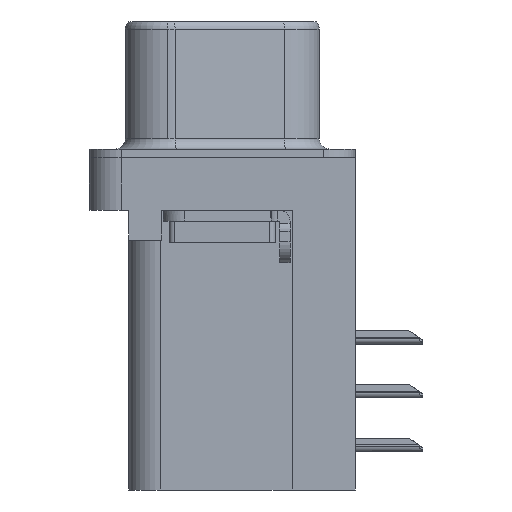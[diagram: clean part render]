
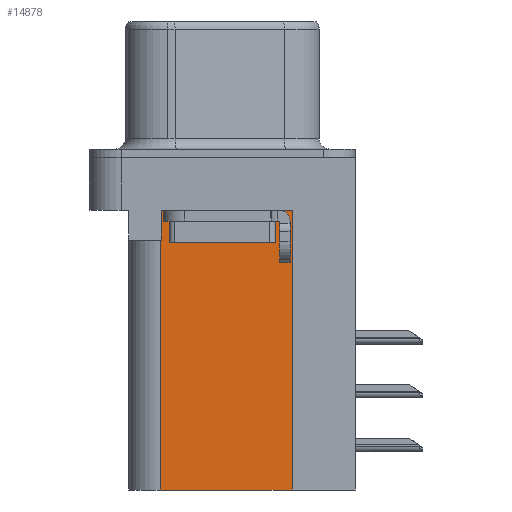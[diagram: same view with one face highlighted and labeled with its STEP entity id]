
A CAD part, left-side view. The second image highlights one B-rep face of the part: STEP entity #14878.
In plain terms, the highlighted planar face has unit normal (-1, 0, 0).
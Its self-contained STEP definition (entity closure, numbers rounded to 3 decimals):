
#390 = CARTESIAN_POINT ( 'NONE',  ( 3.7, -3.295, -15.7 ) ) ;
#563 = CARTESIAN_POINT ( 'NONE',  ( 3.7, -3.295, -15.7 ) ) ;
#1540 = EDGE_CURVE ( 'NONE', #8664, #25485, #20465, .T. ) ;
#1928 = LINE ( 'NONE', #12069, #25458 ) ;
#2034 = ORIENTED_EDGE ( 'NONE', *, *, #10155, .F. ) ;
#2653 = DIRECTION ( 'NONE',  ( 0., 0., -1. ) ) ;
#4221 = ORIENTED_EDGE ( 'NONE', *, *, #1540, .T. ) ;
#5213 = DIRECTION ( 'NONE',  ( 0., 0., 1. ) ) ;
#5603 = EDGE_CURVE ( 'NONE', #20065, #8664, #27021, .T. ) ;
#6796 = LINE ( 'NONE', #17612, #12810 ) ;
#7113 = FACE_OUTER_BOUND ( 'NONE', #16796, .T. ) ;
#8664 = VERTEX_POINT ( 'NONE', #24389 ) ;
#8684 = CARTESIAN_POINT ( 'NONE',  ( 3.7, -3.295, -2.5 ) ) ;
#8689 = DIRECTION ( 'NONE',  ( 0., 1., 0. ) ) ;
#9821 = LINE ( 'NONE', #18837, #22606 ) ;
#10155 = EDGE_CURVE ( 'NONE', #15262, #10890, #9821, .T. ) ;
#10890 = VERTEX_POINT ( 'NONE', #11415 ) ;
#11124 = AXIS2_PLACEMENT_3D ( 'NONE', #390, #16295, #2653 ) ;
#11415 = CARTESIAN_POINT ( 'NONE',  ( 3.7, 2.925, -3.9 ) ) ;
#11631 = CARTESIAN_POINT ( 'NONE',  ( 3.7, 2.895, -3.9 ) ) ;
#12069 = CARTESIAN_POINT ( 'NONE',  ( 3.7, 0., -3.9 ) ) ;
#12181 = EDGE_CURVE ( 'NONE', #12749, #20065, #22903, .T. ) ;
#12749 = VERTEX_POINT ( 'NONE', #28116 ) ;
#12810 = VECTOR ( 'NONE', #20006, 1000. ) ;
#14014 = PLANE ( 'NONE',  #11124 ) ;
#14353 = DIRECTION ( 'NONE',  ( 0., 1., 0. ) ) ;
#14394 = VECTOR ( 'NONE', #25349, 1000. ) ;
#14878 = ADVANCED_FACE ( 'NONE', ( #7113 ), #14014, .F. ) ;
#15262 = VERTEX_POINT ( 'NONE', #19839 ) ;
#16123 = VECTOR ( 'NONE', #25441, 1000. ) ;
#16295 = DIRECTION ( 'NONE',  ( 1., 0., 0. ) ) ;
#16796 = EDGE_LOOP ( 'NONE', ( #21812, #4221, #25150, #2034, #18632, #19967 ) ) ;
#17612 = CARTESIAN_POINT ( 'NONE',  ( 3.7, -3.295, -15.7 ) ) ;
#17690 = CARTESIAN_POINT ( 'NONE',  ( 3.7, -3.295, -2.5 ) ) ;
#18632 = ORIENTED_EDGE ( 'NONE', *, *, #23205, .F. ) ;
#18837 = CARTESIAN_POINT ( 'NONE',  ( 3.7, 2.925, -15.7 ) ) ;
#19839 = CARTESIAN_POINT ( 'NONE',  ( 3.7, 2.925, -15.7 ) ) ;
#19967 = ORIENTED_EDGE ( 'NONE', *, *, #12181, .T. ) ;
#20006 = DIRECTION ( 'NONE',  ( 0., 1., 0. ) ) ;
#20065 = VERTEX_POINT ( 'NONE', #8684 ) ;
#20465 = LINE ( 'NONE', #22916, #14394 ) ;
#20953 = VECTOR ( 'NONE', #8689, 1000. ) ;
#21812 = ORIENTED_EDGE ( 'NONE', *, *, #5603, .T. ) ;
#22606 = VECTOR ( 'NONE', #5213, 1000. ) ;
#22903 = LINE ( 'NONE', #563, #16123 ) ;
#22916 = CARTESIAN_POINT ( 'NONE',  ( 3.7, 2.895, -3.9 ) ) ;
#23205 = EDGE_CURVE ( 'NONE', #12749, #15262, #6796, .T. ) ;
#24389 = CARTESIAN_POINT ( 'NONE',  ( 3.7, 2.895, -2.5 ) ) ;
#25150 = ORIENTED_EDGE ( 'NONE', *, *, #26331, .T. ) ;
#25349 = DIRECTION ( 'NONE',  ( 0., 0., -1. ) ) ;
#25441 = DIRECTION ( 'NONE',  ( 0., 0., 1. ) ) ;
#25458 = VECTOR ( 'NONE', #14353, 1000. ) ;
#25485 = VERTEX_POINT ( 'NONE', #11631 ) ;
#26331 = EDGE_CURVE ( 'NONE', #25485, #10890, #1928, .T. ) ;
#27021 = LINE ( 'NONE', #17690, #20953 ) ;
#28116 = CARTESIAN_POINT ( 'NONE',  ( 3.7, -3.295, -15.7 ) ) ;
